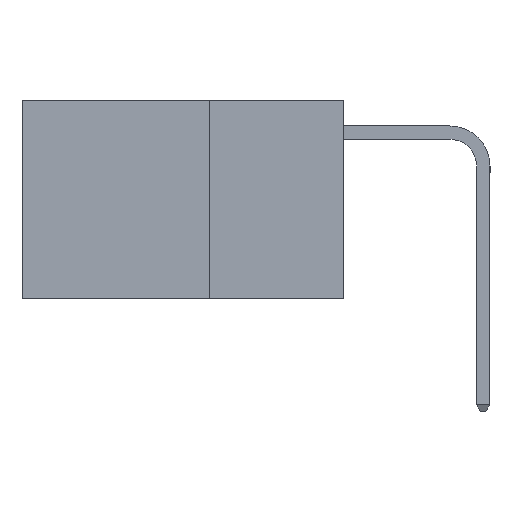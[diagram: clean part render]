
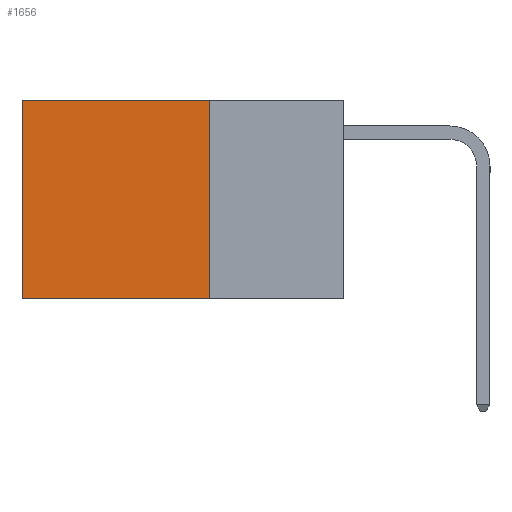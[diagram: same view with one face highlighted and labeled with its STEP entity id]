
A CAD part, left-side view. The second image highlights one B-rep face of the part: STEP entity #1656.
In plain terms, the highlighted planar face has unit normal (-1, 0, 0).
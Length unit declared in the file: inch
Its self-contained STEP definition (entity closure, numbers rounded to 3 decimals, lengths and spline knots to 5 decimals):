
#1656 = ADVANCED_FACE ( 'NONE', ( #11491 ), #4615, .F. ) ;
#2859 = LINE ( 'NONE', #5633, #4907 ) ;
#3897 = VERTEX_POINT ( 'NONE', #10634 ) ;
#4615 = PLANE ( 'NONE',  #9247 ) ;
#4865 = LINE ( 'NONE', #11512, #9379 ) ;
#4907 = VECTOR ( 'NONE', #6531, 39.37008 ) ;
#4912 = VERTEX_POINT ( 'NONE', #5050 ) ;
#5050 = CARTESIAN_POINT ( 'NONE',  ( 0.2625, 0.25, -0.37 ) ) ;
#5453 = DIRECTION ( 'NONE',  ( 0., 0., -1. ) ) ;
#5522 = ORIENTED_EDGE ( 'NONE', *, *, #9665, .T. ) ;
#5532 = ORIENTED_EDGE ( 'NONE', *, *, #8665, .F. ) ;
#5601 = ORIENTED_EDGE ( 'NONE', *, *, #8131, .F. ) ;
#5633 = CARTESIAN_POINT ( 'NONE',  ( 0.2625, 0.25, 0. ) ) ;
#5644 = ORIENTED_EDGE ( 'NONE', *, *, #9978, .T. ) ;
#5893 = VECTOR ( 'NONE', #7936, 39.37008 ) ;
#6047 = VERTEX_POINT ( 'NONE', #6160 ) ;
#6160 = CARTESIAN_POINT ( 'NONE',  ( 0.2625, 0.25, 0. ) ) ;
#6531 = DIRECTION ( 'NONE',  ( 0., 1., 0. ) ) ;
#7028 = DIRECTION ( 'NONE',  ( 1., 0., 0. ) ) ;
#7738 = CARTESIAN_POINT ( 'NONE',  ( 0.2625, 0.25, -0.37 ) ) ;
#7919 = LINE ( 'NONE', #7738, #9679 ) ;
#7936 = DIRECTION ( 'NONE',  ( 0., 0., -1. ) ) ;
#8076 = CARTESIAN_POINT ( 'NONE',  ( 0.2625, 0.6, 0. ) ) ;
#8131 = EDGE_CURVE ( 'NONE', #6047, #4912, #8202, .T. ) ;
#8142 = DIRECTION ( 'NONE',  ( 0., 0., -1. ) ) ;
#8202 = LINE ( 'NONE', #9678, #5893 ) ;
#8665 = EDGE_CURVE ( 'NONE', #4912, #3897, #7919, .T. ) ;
#9247 = AXIS2_PLACEMENT_3D ( 'NONE', #10640, #7028, #5453 ) ;
#9379 = VECTOR ( 'NONE', #8142, 39.37008 ) ;
#9589 = VERTEX_POINT ( 'NONE', #8076 ) ;
#9665 = EDGE_CURVE ( 'NONE', #9589, #3897, #4865, .T. ) ;
#9678 = CARTESIAN_POINT ( 'NONE',  ( 0.2625, 0.25, 0. ) ) ;
#9679 = VECTOR ( 'NONE', #10339, 39.37008 ) ;
#9978 = EDGE_CURVE ( 'NONE', #6047, #9589, #2859, .T. ) ;
#10339 = DIRECTION ( 'NONE',  ( 0., 1., 0. ) ) ;
#10634 = CARTESIAN_POINT ( 'NONE',  ( 0.2625, 0.6, -0.37 ) ) ;
#10640 = CARTESIAN_POINT ( 'NONE',  ( 0.2625, 0.25, 0. ) ) ;
#10698 = EDGE_LOOP ( 'NONE', ( #5522, #5532, #5601, #5644 ) ) ;
#11491 = FACE_OUTER_BOUND ( 'NONE', #10698, .T. ) ;
#11512 = CARTESIAN_POINT ( 'NONE',  ( 0.2625, 0.6, 0. ) ) ;
